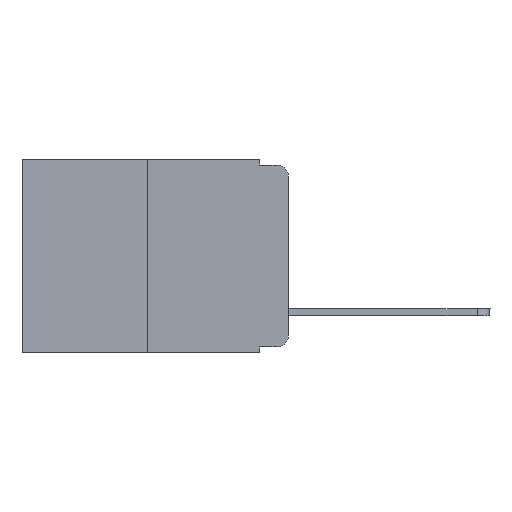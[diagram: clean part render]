
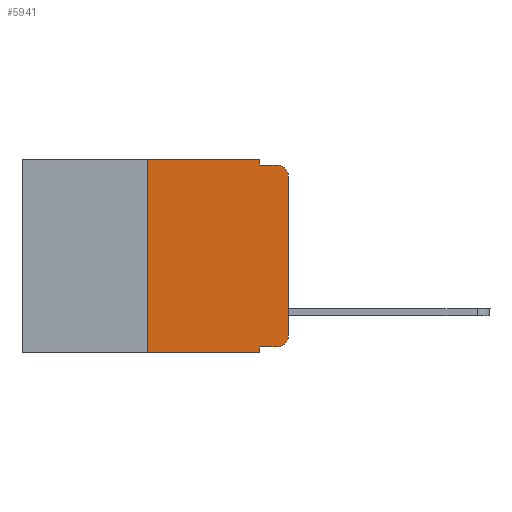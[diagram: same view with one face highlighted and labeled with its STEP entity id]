
A CAD part, left-side view. The second image highlights one B-rep face of the part: STEP entity #5941.
In plain terms, the highlighted planar face has unit normal (-1, 0, 0).
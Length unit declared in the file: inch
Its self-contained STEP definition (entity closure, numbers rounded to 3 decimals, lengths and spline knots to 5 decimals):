
#118 = CIRCLE ( 'NONE', #3370, 0.02 ) ;
#341 = VECTOR ( 'NONE', #10506, 39.37008 ) ;
#364 = ORIENTED_EDGE ( 'NONE', *, *, #7275, .T. ) ;
#893 = DIRECTION ( 'NONE',  ( 0., 0., -1. ) ) ;
#895 = CARTESIAN_POINT ( 'NONE',  ( 0., 0.25, -0.343 ) ) ;
#1043 = VERTEX_POINT ( 'NONE', #11539 ) ;
#1259 = DIRECTION ( 'NONE',  ( 0., 0., 1. ) ) ;
#1401 = CARTESIAN_POINT ( 'NONE',  ( 0., 0.051, -0.333 ) ) ;
#1583 = VERTEX_POINT ( 'NONE', #895 ) ;
#1650 = VECTOR ( 'NONE', #10735, 39.37008 ) ;
#1996 = ORIENTED_EDGE ( 'NONE', *, *, #15256, .F. ) ;
#2178 = EDGE_CURVE ( 'NONE', #3297, #1043, #5830, .T. ) ;
#2296 = ORIENTED_EDGE ( 'NONE', *, *, #13029, .F. ) ;
#2449 = LINE ( 'NONE', #8408, #14347 ) ;
#2529 = VERTEX_POINT ( 'NONE', #11776 ) ;
#2786 = LINE ( 'NONE', #8832, #8047 ) ;
#3171 = CARTESIAN_POINT ( 'NONE',  ( 0., 0.051, 0. ) ) ;
#3297 = VERTEX_POINT ( 'NONE', #3171 ) ;
#3370 = AXIS2_PLACEMENT_3D ( 'NONE', #6923, #4434, #14113 ) ;
#3508 = EDGE_CURVE ( 'NONE', #14260, #7248, #6182, .T. ) ;
#3511 = LINE ( 'NONE', #5532, #341 ) ;
#3735 = LINE ( 'NONE', #10840, #12876 ) ;
#3751 = VECTOR ( 'NONE', #7349, 39.37008 ) ;
#3874 = CARTESIAN_POINT ( 'NONE',  ( 0., 0., 0. ) ) ;
#3977 = CARTESIAN_POINT ( 'NONE',  ( 0., 0., -0.313 ) ) ;
#4043 = VERTEX_POINT ( 'NONE', #12677 ) ;
#4352 = VERTEX_POINT ( 'NONE', #1401 ) ;
#4434 = DIRECTION ( 'NONE',  ( -1., 0., 0. ) ) ;
#4532 = AXIS2_PLACEMENT_3D ( 'NONE', #5736, #12950, #14136 ) ;
#4697 = EDGE_CURVE ( 'NONE', #10018, #3297, #3511, .T. ) ;
#5532 = CARTESIAN_POINT ( 'NONE',  ( 0., 0.473, 0. ) ) ;
#5647 = EDGE_CURVE ( 'NONE', #6294, #4043, #118, .T. ) ;
#5699 = DIRECTION ( 'NONE',  ( 1., 0., 0. ) ) ;
#5736 = CARTESIAN_POINT ( 'NONE',  ( 0., 0.02, -0.313 ) ) ;
#5830 = LINE ( 'NONE', #8639, #3751 ) ;
#5920 = CARTESIAN_POINT ( 'NONE',  ( 0., 0.25, 0. ) ) ;
#5941 = ADVANCED_FACE ( 'NONE', ( #7971 ), #10551, .F. ) ;
#6068 = EDGE_CURVE ( 'NONE', #1583, #10018, #6277, .T. ) ;
#6182 = CIRCLE ( 'NONE', #4532, 0.02 ) ;
#6257 = DIRECTION ( 'NONE',  ( 0., 0., 1. ) ) ;
#6277 = LINE ( 'NONE', #7182, #15370 ) ;
#6294 = VERTEX_POINT ( 'NONE', #12688 ) ;
#6368 = DIRECTION ( 'NONE',  ( 0., -1., 0. ) ) ;
#6621 = ORIENTED_EDGE ( 'NONE', *, *, #9439, .T. ) ;
#6686 = CARTESIAN_POINT ( 'NONE',  ( 0., 0.02, -0.333 ) ) ;
#6923 = CARTESIAN_POINT ( 'NONE',  ( 0., 0.02, -0.03 ) ) ;
#7182 = CARTESIAN_POINT ( 'NONE',  ( 0., 0.25, 0. ) ) ;
#7248 = VERTEX_POINT ( 'NONE', #3977 ) ;
#7275 = EDGE_CURVE ( 'NONE', #7248, #6294, #14566, .T. ) ;
#7349 = DIRECTION ( 'NONE',  ( 0., 0., -1. ) ) ;
#7647 = LINE ( 'NONE', #10933, #1650 ) ;
#7971 = FACE_OUTER_BOUND ( 'NONE', #14606, .T. ) ;
#8047 = VECTOR ( 'NONE', #6368, 39.37008 ) ;
#8145 = ORIENTED_EDGE ( 'NONE', *, *, #3508, .T. ) ;
#8260 = ORIENTED_EDGE ( 'NONE', *, *, #4697, .F. ) ;
#8302 = VECTOR ( 'NONE', #6257, 39.37008 ) ;
#8408 = CARTESIAN_POINT ( 'NONE',  ( 0., 0.051, -0.333 ) ) ;
#8639 = CARTESIAN_POINT ( 'NONE',  ( 0., 0.051, 0. ) ) ;
#8832 = CARTESIAN_POINT ( 'NONE',  ( 0., 0.473, -0.343 ) ) ;
#9059 = EDGE_CURVE ( 'NONE', #1583, #2529, #2786, .T. ) ;
#9439 = EDGE_CURVE ( 'NONE', #4352, #14260, #2449, .T. ) ;
#9694 = ORIENTED_EDGE ( 'NONE', *, *, #2178, .F. ) ;
#10018 = VERTEX_POINT ( 'NONE', #5920 ) ;
#10044 = ORIENTED_EDGE ( 'NONE', *, *, #6068, .F. ) ;
#10506 = DIRECTION ( 'NONE',  ( 0., -1., 0. ) ) ;
#10551 = PLANE ( 'NONE',  #15417 ) ;
#10735 = DIRECTION ( 'NONE',  ( 0., -1., 0. ) ) ;
#10783 = DIRECTION ( 'NONE',  ( 0., -1., 0. ) ) ;
#10840 = CARTESIAN_POINT ( 'NONE',  ( 0., 0.051, 0. ) ) ;
#10933 = CARTESIAN_POINT ( 'NONE',  ( 0., 0.051, -0.01 ) ) ;
#11539 = CARTESIAN_POINT ( 'NONE',  ( 0., 0.051, -0.01 ) ) ;
#11776 = CARTESIAN_POINT ( 'NONE',  ( 0., 0.051, -0.343 ) ) ;
#12677 = CARTESIAN_POINT ( 'NONE',  ( 0., 0.02, -0.01 ) ) ;
#12688 = CARTESIAN_POINT ( 'NONE',  ( 0., 0., -0.03 ) ) ;
#12876 = VECTOR ( 'NONE', #13197, 39.37008 ) ;
#12950 = DIRECTION ( 'NONE',  ( -1., 0., 0. ) ) ;
#13008 = CARTESIAN_POINT ( 'NONE',  ( 0., 0.473, 0. ) ) ;
#13029 = EDGE_CURVE ( 'NONE', #4352, #2529, #3735, .T. ) ;
#13197 = DIRECTION ( 'NONE',  ( 0., 0., -1. ) ) ;
#13537 = ORIENTED_EDGE ( 'NONE', *, *, #9059, .T. ) ;
#14113 = DIRECTION ( 'NONE',  ( 0., 0., -1. ) ) ;
#14136 = DIRECTION ( 'NONE',  ( 0., 0., -1. ) ) ;
#14260 = VERTEX_POINT ( 'NONE', #6686 ) ;
#14347 = VECTOR ( 'NONE', #10783, 39.37008 ) ;
#14440 = ORIENTED_EDGE ( 'NONE', *, *, #5647, .T. ) ;
#14566 = LINE ( 'NONE', #3874, #8302 ) ;
#14606 = EDGE_LOOP ( 'NONE', ( #364, #14440, #1996, #9694, #8260, #10044, #13537, #2296, #6621, #8145 ) ) ;
#15256 = EDGE_CURVE ( 'NONE', #1043, #4043, #7647, .T. ) ;
#15370 = VECTOR ( 'NONE', #1259, 39.37008 ) ;
#15417 = AXIS2_PLACEMENT_3D ( 'NONE', #13008, #5699, #893 ) ;
